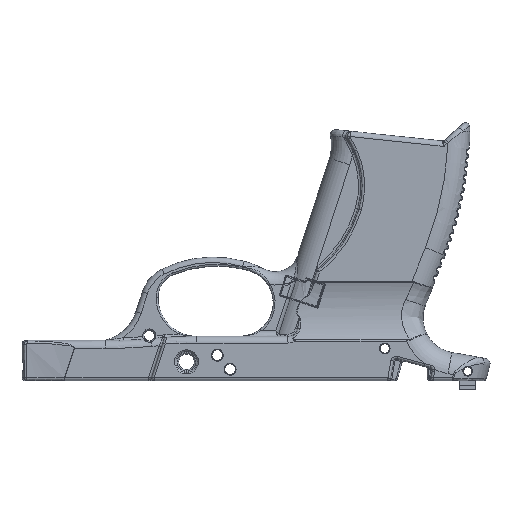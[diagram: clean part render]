
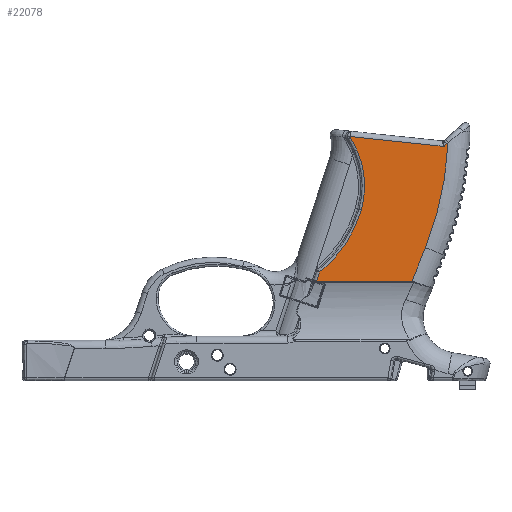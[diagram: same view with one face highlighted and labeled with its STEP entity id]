
A CAD part, front view. The second image highlights one B-rep face of the part: STEP entity #22078.
In plain terms, the highlighted planar face has unit normal (0, -1, 0).
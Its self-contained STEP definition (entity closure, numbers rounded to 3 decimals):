
#880=B_SPLINE_CURVE_WITH_KNOTS('',3,(#43940,#43941,#43942,#43943),
 .UNSPECIFIED.,.F.,.F.,(4,4),(0.,0.039),.UNSPECIFIED.);
#881=B_SPLINE_CURVE_WITH_KNOTS('',3,(#43945,#43946,#43947,#43948),
 .UNSPECIFIED.,.F.,.F.,(4,4),(-1.153,-0.627),
 .UNSPECIFIED.);
#1610=PLANE('',#24097);
#2283=LINE('',#40081,#3369);
#2463=LINE('',#43904,#3549);
#2466=LINE('',#43929,#3552);
#2467=LINE('',#43932,#3553);
#2468=LINE('',#43934,#3554);
#2469=LINE('',#43938,#3555);
#3369=VECTOR('',#27430,10.);
#3549=VECTOR('',#28394,10.);
#3552=VECTOR('',#28409,10.);
#3553=VECTOR('',#28414,10.);
#3554=VECTOR('',#28415,10.);
#3555=VECTOR('',#28418,10.);
#5207=FACE_OUTER_BOUND('',#6702,.T.);
#6702=EDGE_LOOP('',(#17387,#17388,#17389,#17390,#17391,#17392,#17393,#17394,
#17395,#17396,#17397,#17398));
#7959=CIRCLE('',#23616,120.212);
#8199=CIRCLE('',#24098,8.5);
#8200=CIRCLE('',#24099,32.518);
#8201=CIRCLE('',#24100,45.518);
#9650=VERTEX_POINT('',#38637);
#9651=VERTEX_POINT('',#38643);
#9727=VERTEX_POINT('',#40080);
#10040=VERTEX_POINT('',#43854);
#10041=VERTEX_POINT('',#43877);
#10048=VERTEX_POINT('',#43928);
#10049=VERTEX_POINT('',#43933);
#10050=VERTEX_POINT('',#43935);
#10051=VERTEX_POINT('',#43937);
#10052=VERTEX_POINT('',#43939);
#10053=VERTEX_POINT('',#43944);
#10054=VERTEX_POINT('',#43949);
#11938=EDGE_CURVE('',#9650,#9651,#7959,.T.);
#12073=EDGE_CURVE('',#9651,#9727,#2283,.T.);
#12611=EDGE_CURVE('',#10041,#10040,#2463,.T.);
#12619=EDGE_CURVE('',#10040,#10048,#2466,.T.);
#12621=EDGE_CURVE('',#9727,#10041,#2467,.T.);
#12622=EDGE_CURVE('',#10049,#9650,#2468,.T.);
#12623=EDGE_CURVE('',#10050,#10049,#8199,.T.);
#12624=EDGE_CURVE('',#10051,#10050,#2469,.T.);
#12625=EDGE_CURVE('',#10052,#10051,#880,.T.);
#12626=EDGE_CURVE('',#10053,#10052,#881,.T.);
#12627=EDGE_CURVE('',#10054,#10053,#8200,.T.);
#12628=EDGE_CURVE('',#10048,#10054,#8201,.T.);
#17387=ORIENTED_EDGE('',*,*,#12611,.F.);
#17388=ORIENTED_EDGE('',*,*,#12621,.F.);
#17389=ORIENTED_EDGE('',*,*,#12073,.F.);
#17390=ORIENTED_EDGE('',*,*,#11938,.F.);
#17391=ORIENTED_EDGE('',*,*,#12622,.F.);
#17392=ORIENTED_EDGE('',*,*,#12623,.F.);
#17393=ORIENTED_EDGE('',*,*,#12624,.F.);
#17394=ORIENTED_EDGE('',*,*,#12625,.F.);
#17395=ORIENTED_EDGE('',*,*,#12626,.F.);
#17396=ORIENTED_EDGE('',*,*,#12627,.F.);
#17397=ORIENTED_EDGE('',*,*,#12628,.F.);
#17398=ORIENTED_EDGE('',*,*,#12619,.F.);
#22078=ADVANCED_FACE('',(#5207),#1610,.T.);
#23616=AXIS2_PLACEMENT_3D('',#38644,#27230,#27231);
#24097=AXIS2_PLACEMENT_3D('',#43931,#28412,#28413);
#24098=AXIS2_PLACEMENT_3D('',#43936,#28416,#28417);
#24099=AXIS2_PLACEMENT_3D('',#43950,#28419,#28420);
#24100=AXIS2_PLACEMENT_3D('',#43951,#28421,#28422);
#27230=DIRECTION('center_axis',(0.,1.,0.));
#27231=DIRECTION('ref_axis',(0.981,0.,-0.194));
#27430=DIRECTION('',(-0.371,0.,-0.929));
#28394=DIRECTION('',(-0.952,0.,0.306));
#28409=DIRECTION('',(0.309,0.,0.951));
#28412=DIRECTION('center_axis',(0.,-1.,0.));
#28413=DIRECTION('ref_axis',(1.,0.,0.));
#28414=DIRECTION('',(-1.,0.,0.));
#28415=DIRECTION('',(0.741,0.,0.672));
#28416=DIRECTION('center_axis',(0.,1.,0.));
#28417=DIRECTION('ref_axis',(-0.758,0.,0.652));
#28418=DIRECTION('',(0.995,0.,-0.105));
#28419=DIRECTION('center_axis',(0.,-1.,0.));
#28420=DIRECTION('ref_axis',(0.997,0.,0.072));
#28421=DIRECTION('center_axis',(0.,-1.,0.));
#28422=DIRECTION('ref_axis',(0.835,0.,-0.551));
#38637=CARTESIAN_POINT('',(83.026,-13.75,48.883));
#38643=CARTESIAN_POINT('',(74.571,-13.75,9.633));
#38644=CARTESIAN_POINT('Origin',(-37.068,-13.75,54.219));
#40080=CARTESIAN_POINT('',(69.538,-13.75,-2.968));
#40081=CARTESIAN_POINT('',(76.221,-13.75,13.765));
#43854=CARTESIAN_POINT('',(33.966,-13.75,-2.917));
#43877=CARTESIAN_POINT('',(34.126,-13.75,-2.968));
#43904=CARTESIAN_POINT('',(38.447,-13.75,-4.356));
#43928=CARTESIAN_POINT('',(35.084,-13.75,0.524));
#43929=CARTESIAN_POINT('',(35.776,-13.75,2.654));
#43931=CARTESIAN_POINT('Origin',(59.201,-13.75,25.354));
#43932=CARTESIAN_POINT('',(110.,-13.75,-2.968));
#43933=CARTESIAN_POINT('',(82.421,-13.75,48.334));
#43934=CARTESIAN_POINT('',(69.981,-13.75,37.054));
#43935=CARTESIAN_POINT('',(81.522,-13.75,47.383));
#43936=CARTESIAN_POINT('Origin',(88.13,-13.75,42.037));
#43937=CARTESIAN_POINT('',(46.455,-13.75,51.069));
#43938=CARTESIAN_POINT('',(49.586,-13.75,50.74));
#43939=CARTESIAN_POINT('',(46.545,-13.75,50.692));
#43940=CARTESIAN_POINT('Ctrl Pts',(46.545,-13.75,50.692));
#43941=CARTESIAN_POINT('Ctrl Pts',(46.477,-13.75,50.805));
#43942=CARTESIAN_POINT('Ctrl Pts',(46.441,-13.75,50.938));
#43943=CARTESIAN_POINT('Ctrl Pts',(46.455,-13.75,51.069));
#43944=CARTESIAN_POINT('',(48.99,-13.75,46.038));
#43945=CARTESIAN_POINT('Ctrl Pts',(48.99,-13.75,46.038));
#43946=CARTESIAN_POINT('Ctrl Pts',(48.267,-13.75,47.636));
#43947=CARTESIAN_POINT('Ctrl Pts',(47.451,-13.75,49.191));
#43948=CARTESIAN_POINT('Ctrl Pts',(46.545,-13.75,50.692));
#43949=CARTESIAN_POINT('',(50.603,-13.75,23.613));
#43950=CARTESIAN_POINT('Origin',(19.362,-13.75,32.637));
#43951=CARTESIAN_POINT('Origin',(6.873,-13.75,36.245));
